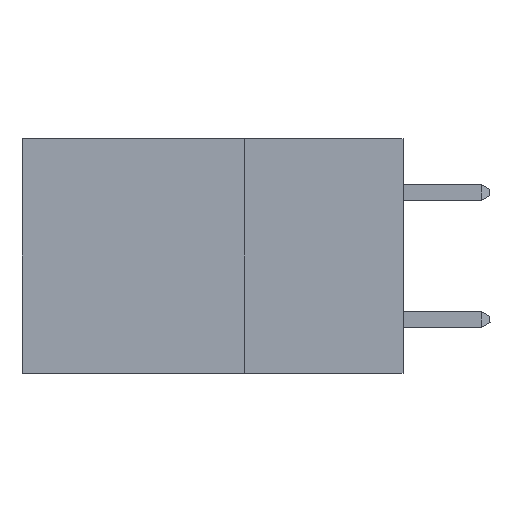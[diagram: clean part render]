
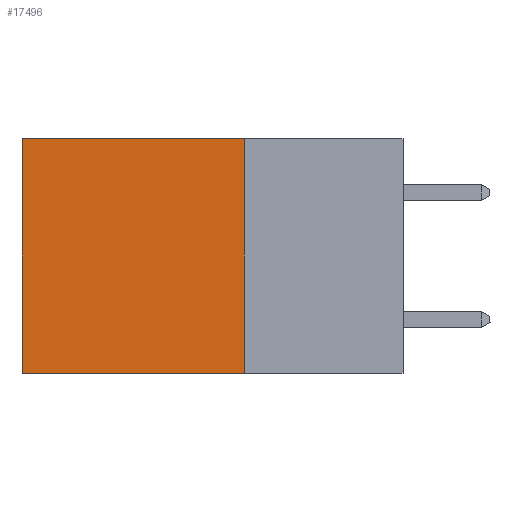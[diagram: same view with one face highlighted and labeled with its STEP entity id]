
A CAD part, left-side view. The second image highlights one B-rep face of the part: STEP entity #17496.
In plain terms, the highlighted planar face has unit normal (-1, 0, 0).
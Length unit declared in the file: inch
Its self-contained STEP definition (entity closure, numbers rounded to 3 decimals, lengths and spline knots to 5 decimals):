
#374 = CARTESIAN_POINT ( 'NONE',  ( 0.2875, 0.25, -0.37 ) ) ;
#1241 = VECTOR ( 'NONE', #22147, 39.37008 ) ;
#1686 = CARTESIAN_POINT ( 'NONE',  ( 0.2875, 0.25, 0. ) ) ;
#1888 = CARTESIAN_POINT ( 'NONE',  ( 0.2875, 0.6, -0.37 ) ) ;
#2318 = CARTESIAN_POINT ( 'NONE',  ( 0.2875, 0.25, 0. ) ) ;
#2720 = VERTEX_POINT ( 'NONE', #21040 ) ;
#3932 = LINE ( 'NONE', #22028, #38092 ) ;
#5752 = DIRECTION ( 'NONE',  ( 0., 0., -1. ) ) ;
#11211 = EDGE_CURVE ( 'NONE', #43920, #28234, #17257, .T. ) ;
#12179 = CARTESIAN_POINT ( 'NONE',  ( 0.2875, 0.6, 0. ) ) ;
#14243 = ORIENTED_EDGE ( 'NONE', *, *, #38346, .F. ) ;
#15125 = DIRECTION ( 'NONE',  ( 0., 0., -1. ) ) ;
#15626 = CARTESIAN_POINT ( 'NONE',  ( 0.2875, 0.6, 0. ) ) ;
#17257 = LINE ( 'NONE', #1686, #1241 ) ;
#17496 = ADVANCED_FACE ( 'NONE', ( #22456 ), #29549, .F. ) ;
#19210 = AXIS2_PLACEMENT_3D ( 'NONE', #2318, #26272, #5752 ) ;
#20200 = ORIENTED_EDGE ( 'NONE', *, *, #41740, .F. ) ;
#21040 = CARTESIAN_POINT ( 'NONE',  ( 0.2875, 0.25, -0.37 ) ) ;
#21240 = CARTESIAN_POINT ( 'NONE',  ( 0.2875, 0.25, 0. ) ) ;
#21979 = VECTOR ( 'NONE', #36063, 39.37008 ) ;
#22028 = CARTESIAN_POINT ( 'NONE',  ( 0.2875, 0.25, 0. ) ) ;
#22147 = DIRECTION ( 'NONE',  ( 0., 1., 0. ) ) ;
#22456 = FACE_OUTER_BOUND ( 'NONE', #38167, .T. ) ;
#24103 = ORIENTED_EDGE ( 'NONE', *, *, #11211, .T. ) ;
#24336 = DIRECTION ( 'NONE',  ( 0., 1., 0. ) ) ;
#26272 = DIRECTION ( 'NONE',  ( 1., 0., 0. ) ) ;
#27166 = LINE ( 'NONE', #374, #36152 ) ;
#28234 = VERTEX_POINT ( 'NONE', #15626 ) ;
#28867 = VERTEX_POINT ( 'NONE', #1888 ) ;
#29549 = PLANE ( 'NONE',  #19210 ) ;
#30041 = LINE ( 'NONE', #12179, #21979 ) ;
#31433 = EDGE_CURVE ( 'NONE', #28234, #28867, #30041, .T. ) ;
#36063 = DIRECTION ( 'NONE',  ( 0., 0., -1. ) ) ;
#36152 = VECTOR ( 'NONE', #24336, 39.37008 ) ;
#37866 = ORIENTED_EDGE ( 'NONE', *, *, #31433, .T. ) ;
#38092 = VECTOR ( 'NONE', #15125, 39.37008 ) ;
#38167 = EDGE_LOOP ( 'NONE', ( #37866, #20200, #14243, #24103 ) ) ;
#38346 = EDGE_CURVE ( 'NONE', #43920, #2720, #3932, .T. ) ;
#41740 = EDGE_CURVE ( 'NONE', #2720, #28867, #27166, .T. ) ;
#43920 = VERTEX_POINT ( 'NONE', #21240 ) ;
